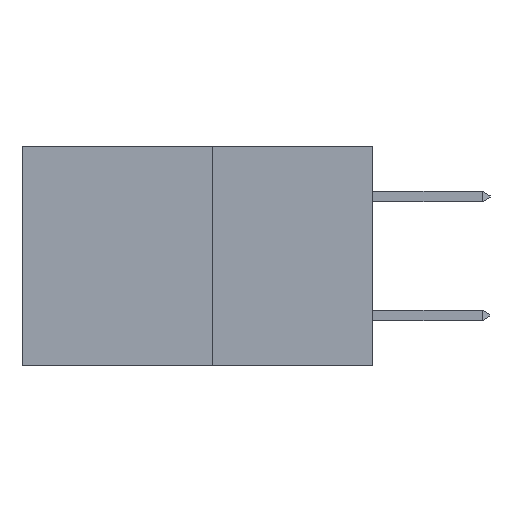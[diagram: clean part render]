
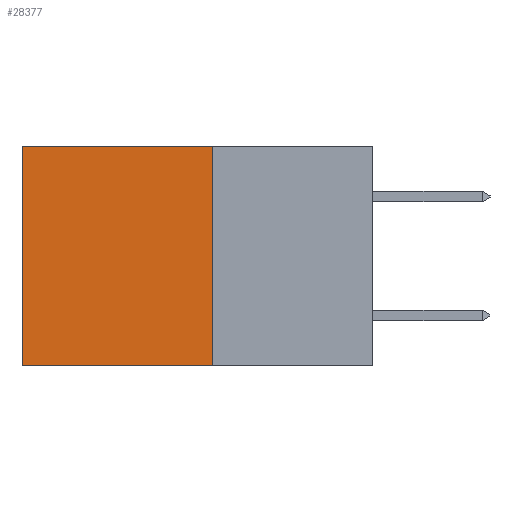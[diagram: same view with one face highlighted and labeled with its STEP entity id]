
A CAD part, left-side view. The second image highlights one B-rep face of the part: STEP entity #28377.
In plain terms, the highlighted planar face has unit normal (-1, 0, 0).
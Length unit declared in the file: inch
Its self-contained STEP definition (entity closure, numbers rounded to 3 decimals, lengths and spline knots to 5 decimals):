
#3440 = VECTOR ( 'NONE', #5506, 39.37008 ) ;
#4901 = EDGE_CURVE ( 'NONE', #27019, #32739, #22903, .T. ) ;
#4979 = CARTESIAN_POINT ( 'NONE',  ( 0.277, 0.59, -0.37 ) ) ;
#5506 = DIRECTION ( 'NONE',  ( 0., 0., -1. ) ) ;
#6090 = CARTESIAN_POINT ( 'NONE',  ( 0.277, 0.27, -0.37 ) ) ;
#6196 = ORIENTED_EDGE ( 'NONE', *, *, #20233, .F. ) ;
#6732 = CARTESIAN_POINT ( 'NONE',  ( 0.277, 0.27, 0. ) ) ;
#6990 = VERTEX_POINT ( 'NONE', #4979 ) ;
#7227 = DIRECTION ( 'NONE',  ( 1., 0., 0. ) ) ;
#11389 = VECTOR ( 'NONE', #20549, 39.37008 ) ;
#12039 = ORIENTED_EDGE ( 'NONE', *, *, #13778, .T. ) ;
#13020 = CARTESIAN_POINT ( 'NONE',  ( 0.277, 0.59, -0.37 ) ) ;
#13214 = CARTESIAN_POINT ( 'NONE',  ( 0.277, 0.27, -0.37 ) ) ;
#13710 = FACE_OUTER_BOUND ( 'NONE', #26494, .T. ) ;
#13778 = EDGE_CURVE ( 'NONE', #28809, #6990, #30764, .T. ) ;
#14618 = ORIENTED_EDGE ( 'NONE', *, *, #4901, .F. ) ;
#15312 = DIRECTION ( 'NONE',  ( 0., 1., 0. ) ) ;
#19476 = ORIENTED_EDGE ( 'NONE', *, *, #20704, .T. ) ;
#20233 = EDGE_CURVE ( 'NONE', #32739, #6990, #30050, .T. ) ;
#20524 = AXIS2_PLACEMENT_3D ( 'NONE', #32402, #7227, #24921 ) ;
#20549 = DIRECTION ( 'NONE',  ( 0., 0., -1. ) ) ;
#20704 = EDGE_CURVE ( 'NONE', #27019, #28809, #30023, .T. ) ;
#20852 = DIRECTION ( 'NONE',  ( 0., 1., 0. ) ) ;
#22375 = PLANE ( 'NONE',  #20524 ) ;
#22524 = VECTOR ( 'NONE', #15312, 39.37008 ) ;
#22903 = LINE ( 'NONE', #6090, #3440 ) ;
#24921 = DIRECTION ( 'NONE',  ( 0., 0., -1. ) ) ;
#26460 = CARTESIAN_POINT ( 'NONE',  ( 0.277, 0.59, 0. ) ) ;
#26494 = EDGE_LOOP ( 'NONE', ( #12039, #6196, #14618, #19476 ) ) ;
#27019 = VERTEX_POINT ( 'NONE', #6732 ) ;
#27926 = CARTESIAN_POINT ( 'NONE',  ( 0.277, 0.27, 0. ) ) ;
#28377 = ADVANCED_FACE ( 'NONE', ( #13710 ), #22375, .F. ) ;
#28809 = VERTEX_POINT ( 'NONE', #26460 ) ;
#28820 = CARTESIAN_POINT ( 'NONE',  ( 0.277, 0.27, -0.37 ) ) ;
#29282 = VECTOR ( 'NONE', #20852, 39.37008 ) ;
#30023 = LINE ( 'NONE', #27926, #22524 ) ;
#30050 = LINE ( 'NONE', #13214, #29282 ) ;
#30764 = LINE ( 'NONE', #13020, #11389 ) ;
#32402 = CARTESIAN_POINT ( 'NONE',  ( 0.277, 0.27, -0.37 ) ) ;
#32739 = VERTEX_POINT ( 'NONE', #28820 ) ;
